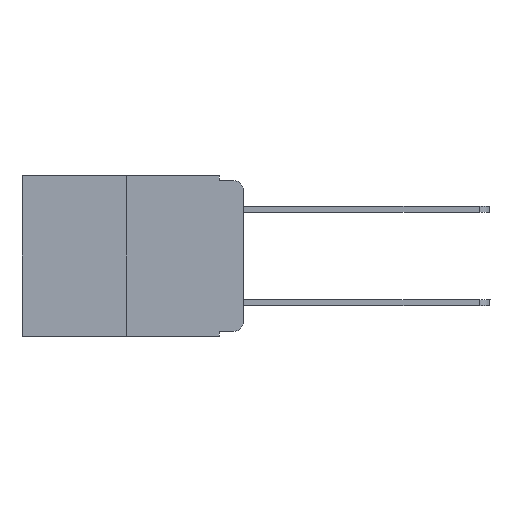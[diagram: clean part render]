
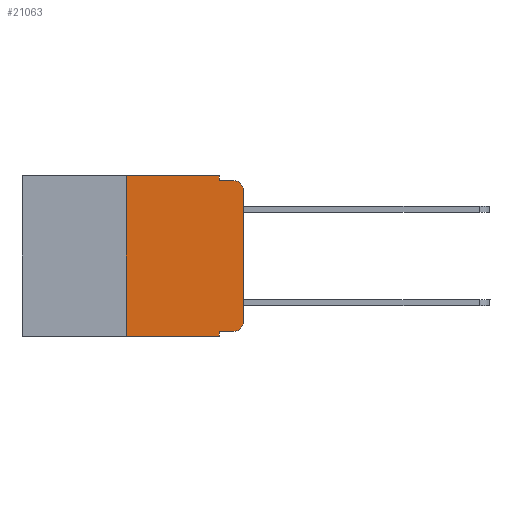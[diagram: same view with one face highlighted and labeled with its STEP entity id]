
A CAD part, left-side view. The second image highlights one B-rep face of the part: STEP entity #21063.
In plain terms, the highlighted planar face has unit normal (-1, 0, 0).
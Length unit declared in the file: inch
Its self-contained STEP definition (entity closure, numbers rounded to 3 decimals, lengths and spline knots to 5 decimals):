
#256 = ORIENTED_EDGE ( 'NONE', *, *, #14406, .T. ) ;
#668 = DIRECTION ( 'NONE',  ( 0., 0., -1. ) ) ;
#800 = EDGE_CURVE ( 'NONE', #4875, #9216, #23070, .T. ) ;
#1459 = CARTESIAN_POINT ( 'NONE',  ( 0., 0.02, -0.333 ) ) ;
#1759 = ORIENTED_EDGE ( 'NONE', *, *, #6827, .T. ) ;
#2260 = ORIENTED_EDGE ( 'NONE', *, *, #7755, .F. ) ;
#2583 = DIRECTION ( 'NONE',  ( 0., 0., -1. ) ) ;
#3126 = CARTESIAN_POINT ( 'NONE',  ( 0., 0.051, -0.333 ) ) ;
#3210 = CIRCLE ( 'NONE', #9563, 0.02 ) ;
#3244 = DIRECTION ( 'NONE',  ( 0., -1., 0. ) ) ;
#3503 = DIRECTION ( 'NONE',  ( 0., 0., 1. ) ) ;
#3509 = EDGE_CURVE ( 'NONE', #21616, #5154, #22277, .T. ) ;
#4454 = CARTESIAN_POINT ( 'NONE',  ( 0., 0.02, -0.01 ) ) ;
#4769 = CARTESIAN_POINT ( 'NONE',  ( 0., 0.051, -0.333 ) ) ;
#4875 = VERTEX_POINT ( 'NONE', #5696 ) ;
#5154 = VERTEX_POINT ( 'NONE', #1459 ) ;
#5258 = CARTESIAN_POINT ( 'NONE',  ( 0., 0.02, -0.03 ) ) ;
#5272 = AXIS2_PLACEMENT_3D ( 'NONE', #23700, #19672, #668 ) ;
#5669 = VERTEX_POINT ( 'NONE', #6670 ) ;
#5696 = CARTESIAN_POINT ( 'NONE',  ( 0., 0.051, -0.01 ) ) ;
#5907 = DIRECTION ( 'NONE',  ( 0., -1., 0. ) ) ;
#6422 = DIRECTION ( 'NONE',  ( -1., 0., 0. ) ) ;
#6432 = EDGE_CURVE ( 'NONE', #20819, #5669, #21623, .T. ) ;
#6521 = LINE ( 'NONE', #14143, #23896 ) ;
#6670 = CARTESIAN_POINT ( 'NONE',  ( 0., 0., -0.03 ) ) ;
#6802 = ORIENTED_EDGE ( 'NONE', *, *, #21649, .F. ) ;
#6827 = EDGE_CURVE ( 'NONE', #5154, #20819, #18697, .T. ) ;
#6914 = ORIENTED_EDGE ( 'NONE', *, *, #8434, .F. ) ;
#7084 = CARTESIAN_POINT ( 'NONE',  ( 0., 0., -0.313 ) ) ;
#7201 = DIRECTION ( 'NONE',  ( 0., 0., -1. ) ) ;
#7554 = CARTESIAN_POINT ( 'NONE',  ( 0., 0.051, 0. ) ) ;
#7660 = ORIENTED_EDGE ( 'NONE', *, *, #800, .F. ) ;
#7678 = EDGE_CURVE ( 'NONE', #21616, #8801, #22619, .T. ) ;
#7755 = EDGE_CURVE ( 'NONE', #13913, #4875, #17078, .T. ) ;
#7935 = VECTOR ( 'NONE', #7201, 39.37008 ) ;
#8434 = EDGE_CURVE ( 'NONE', #11600, #13913, #6521, .T. ) ;
#8801 = VERTEX_POINT ( 'NONE', #21387 ) ;
#8988 = LINE ( 'NONE', #20511, #9270 ) ;
#9216 = VERTEX_POINT ( 'NONE', #4454 ) ;
#9270 = VECTOR ( 'NONE', #3503, 39.37008 ) ;
#9563 = AXIS2_PLACEMENT_3D ( 'NONE', #5258, #20280, #16389 ) ;
#10241 = ORIENTED_EDGE ( 'NONE', *, *, #6432, .T. ) ;
#10411 = VECTOR ( 'NONE', #22943, 39.37008 ) ;
#10985 = EDGE_CURVE ( 'NONE', #19132, #8801, #23080, .T. ) ;
#11139 = ORIENTED_EDGE ( 'NONE', *, *, #10985, .T. ) ;
#11182 = CARTESIAN_POINT ( 'NONE',  ( 0., 0.051, 0. ) ) ;
#11283 = VECTOR ( 'NONE', #5907, 39.37008 ) ;
#11600 = VERTEX_POINT ( 'NONE', #18276 ) ;
#11887 = CARTESIAN_POINT ( 'NONE',  ( 0., 0.25, -0.343 ) ) ;
#12383 = DIRECTION ( 'NONE',  ( 0., -1., 0. ) ) ;
#13913 = VERTEX_POINT ( 'NONE', #16543 ) ;
#14140 = VECTOR ( 'NONE', #3244, 39.37008 ) ;
#14143 = CARTESIAN_POINT ( 'NONE',  ( 0., 0.473, 0. ) ) ;
#14406 = EDGE_CURVE ( 'NONE', #5669, #9216, #3210, .T. ) ;
#15275 = CARTESIAN_POINT ( 'NONE',  ( 0., 0.051, -0.01 ) ) ;
#15800 = CARTESIAN_POINT ( 'NONE',  ( 0., 0.473, -0.343 ) ) ;
#16034 = PLANE ( 'NONE',  #5272 ) ;
#16389 = DIRECTION ( 'NONE',  ( 0., 0., -1. ) ) ;
#16543 = CARTESIAN_POINT ( 'NONE',  ( 0., 0.051, 0. ) ) ;
#16704 = VECTOR ( 'NONE', #23500, 39.37008 ) ;
#17078 = LINE ( 'NONE', #11182, #22358 ) ;
#18276 = CARTESIAN_POINT ( 'NONE',  ( 0., 0.25, 0. ) ) ;
#18697 = CIRCLE ( 'NONE', #19083, 0.02 ) ;
#19083 = AXIS2_PLACEMENT_3D ( 'NONE', #19585, #6422, #2583 ) ;
#19132 = VERTEX_POINT ( 'NONE', #11887 ) ;
#19585 = CARTESIAN_POINT ( 'NONE',  ( 0., 0.02, -0.313 ) ) ;
#19672 = DIRECTION ( 'NONE',  ( 1., 0., 0. ) ) ;
#20182 = FACE_OUTER_BOUND ( 'NONE', #20705, .T. ) ;
#20280 = DIRECTION ( 'NONE',  ( -1., 0., 0. ) ) ;
#20511 = CARTESIAN_POINT ( 'NONE',  ( 0., 0.25, 0. ) ) ;
#20705 = EDGE_LOOP ( 'NONE', ( #10241, #256, #7660, #2260, #6914, #6802, #11139, #24597, #20799, #1759 ) ) ;
#20799 = ORIENTED_EDGE ( 'NONE', *, *, #3509, .T. ) ;
#20819 = VERTEX_POINT ( 'NONE', #7084 ) ;
#21063 = ADVANCED_FACE ( 'NONE', ( #20182 ), #16034, .F. ) ;
#21387 = CARTESIAN_POINT ( 'NONE',  ( 0., 0.051, -0.343 ) ) ;
#21503 = CARTESIAN_POINT ( 'NONE',  ( 0., 0., 0. ) ) ;
#21616 = VERTEX_POINT ( 'NONE', #4769 ) ;
#21623 = LINE ( 'NONE', #21503, #16704 ) ;
#21649 = EDGE_CURVE ( 'NONE', #19132, #11600, #8988, .T. ) ;
#22277 = LINE ( 'NONE', #3126, #14140 ) ;
#22358 = VECTOR ( 'NONE', #24613, 39.37008 ) ;
#22619 = LINE ( 'NONE', #7554, #7935 ) ;
#22943 = DIRECTION ( 'NONE',  ( 0., -1., 0. ) ) ;
#23070 = LINE ( 'NONE', #15275, #10411 ) ;
#23080 = LINE ( 'NONE', #15800, #11283 ) ;
#23500 = DIRECTION ( 'NONE',  ( 0., 0., 1. ) ) ;
#23700 = CARTESIAN_POINT ( 'NONE',  ( 0., 0.473, 0. ) ) ;
#23896 = VECTOR ( 'NONE', #12383, 39.37008 ) ;
#24597 = ORIENTED_EDGE ( 'NONE', *, *, #7678, .F. ) ;
#24613 = DIRECTION ( 'NONE',  ( 0., 0., -1. ) ) ;
